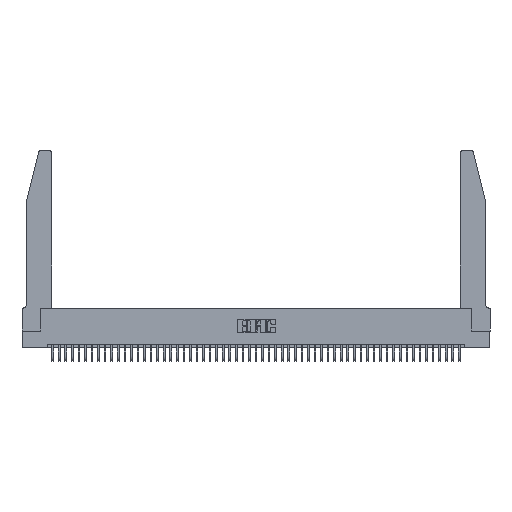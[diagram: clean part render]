
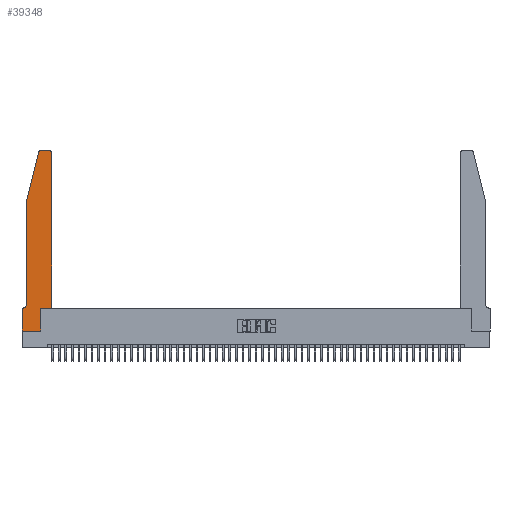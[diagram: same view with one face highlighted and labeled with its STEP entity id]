
A CAD part, top view. The second image highlights one B-rep face of the part: STEP entity #39348.
In plain terms, the highlighted planar face has unit normal (0, 0, 1).
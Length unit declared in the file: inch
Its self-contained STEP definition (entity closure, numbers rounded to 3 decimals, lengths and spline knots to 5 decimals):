
#161 = LINE ( 'NONE', #11159, #33100 ) ;
#1944 = AXIS2_PLACEMENT_3D ( 'NONE', #32347, #7744, #36463 ) ;
#1962 = CARTESIAN_POINT ( 'NONE',  ( 0.0755, 0.35, 0.37 ) ) ;
#2098 = ORIENTED_EDGE ( 'NONE', *, *, #39036, .T. ) ;
#2724 = VECTOR ( 'NONE', #28779, 39.37008 ) ;
#3052 = CARTESIAN_POINT ( 'NONE',  ( 0.25487, 2.72718, 0.37 ) ) ;
#3639 = ORIENTED_EDGE ( 'NONE', *, *, #39453, .T. ) ;
#4787 = EDGE_CURVE ( 'NONE', #17906, #26428, #24658, .T. ) ;
#5095 = VECTOR ( 'NONE', #18629, 39.37008 ) ;
#5466 = CARTESIAN_POINT ( 'NONE',  ( 0.2865, 0.35, 0.37 ) ) ;
#5664 = VERTEX_POINT ( 'NONE', #5466 ) ;
#6022 = CARTESIAN_POINT ( 'NONE',  ( 0.4505, 0.35, 0.37 ) ) ;
#6706 = EDGE_CURVE ( 'NONE', #15442, #36207, #12952, .T. ) ;
#7058 = ORIENTED_EDGE ( 'NONE', *, *, #6706, .T. ) ;
#7272 = EDGE_CURVE ( 'NONE', #49576, #31790, #52472, .T. ) ;
#7744 = DIRECTION ( 'NONE',  ( 0., 0., 1. ) ) ;
#7848 = VERTEX_POINT ( 'NONE', #42641 ) ;
#8058 = CARTESIAN_POINT ( 'NONE',  ( 0.0755, 2., 0.37 ) ) ;
#8470 = CARTESIAN_POINT ( 'NONE',  ( 0., 0.35, 0.37 ) ) ;
#10152 = DIRECTION ( 'NONE',  ( -1., 0., 0. ) ) ;
#10817 = CARTESIAN_POINT ( 'NONE',  ( 0.4205, 2.72, 0.37 ) ) ;
#11159 = CARTESIAN_POINT ( 'NONE',  ( 0., 0., 0.37 ) ) ;
#12011 = CARTESIAN_POINT ( 'NONE',  ( 0.2605, 2.75, 0.37 ) ) ;
#12945 = VERTEX_POINT ( 'NONE', #38376 ) ;
#12949 = FACE_OUTER_BOUND ( 'NONE', #35322, .T. ) ;
#12952 = CIRCLE ( 'NONE', #1944, 0.03 ) ;
#13462 = DIRECTION ( 'NONE',  ( 0., 0., -1. ) ) ;
#13752 = VECTOR ( 'NONE', #10152, 39.37008 ) ;
#14479 = CARTESIAN_POINT ( 'NONE',  ( 0.4505, 0.35, 0.37 ) ) ;
#14942 = DIRECTION ( 'NONE',  ( 1., 0., 0. ) ) ;
#14978 = CARTESIAN_POINT ( 'NONE',  ( 0.0755, 0.42, 0.37 ) ) ;
#15179 = VERTEX_POINT ( 'NONE', #40753 ) ;
#15194 = EDGE_CURVE ( 'NONE', #15179, #7848, #45308, .T. ) ;
#15442 = VERTEX_POINT ( 'NONE', #46208 ) ;
#15621 = ORIENTED_EDGE ( 'NONE', *, *, #24642, .T. ) ;
#16745 = DIRECTION ( 'NONE',  ( 0., 0., 1. ) ) ;
#16920 = VECTOR ( 'NONE', #31723, 39.37008 ) ;
#17074 = CARTESIAN_POINT ( 'NONE',  ( 0.4505, 0.35, 0.37 ) ) ;
#17879 = EDGE_CURVE ( 'NONE', #12945, #15442, #19549, .T. ) ;
#17906 = VERTEX_POINT ( 'NONE', #8058 ) ;
#18629 = DIRECTION ( 'NONE',  ( 1., 0., 0. ) ) ;
#19549 = LINE ( 'NONE', #12011, #50748 ) ;
#21820 = ORIENTED_EDGE ( 'NONE', *, *, #4787, .T. ) ;
#23249 = VERTEX_POINT ( 'NONE', #42673 ) ;
#23628 = VECTOR ( 'NONE', #32767, 39.37008 ) ;
#24642 = EDGE_CURVE ( 'NONE', #23249, #5664, #49626, .T. ) ;
#24658 = LINE ( 'NONE', #48991, #2724 ) ;
#24697 = LINE ( 'NONE', #1962, #13752 ) ;
#25936 = ORIENTED_EDGE ( 'NONE', *, *, #42427, .T. ) ;
#26428 = VERTEX_POINT ( 'NONE', #14978 ) ;
#26989 = LINE ( 'NONE', #14479, #5095 ) ;
#27139 = CIRCLE ( 'NONE', #40269, 0.03 ) ;
#27840 = LINE ( 'NONE', #39721, #16920 ) ;
#28653 = CARTESIAN_POINT ( 'NONE',  ( 0., 0., 0.37 ) ) ;
#28666 = CARTESIAN_POINT ( 'NONE',  ( 0.4505, 2.72, 0.37 ) ) ;
#28779 = DIRECTION ( 'NONE',  ( 0., -1., 0. ) ) ;
#31723 = DIRECTION ( 'NONE',  ( -0.239, -0.971, 0. ) ) ;
#31790 = VERTEX_POINT ( 'NONE', #28666 ) ;
#32347 = CARTESIAN_POINT ( 'NONE',  ( 0.284, 2.72, 0.37 ) ) ;
#32767 = DIRECTION ( 'NONE',  ( 0., -1., 0. ) ) ;
#32853 = ORIENTED_EDGE ( 'NONE', *, *, #49271, .T. ) ;
#33100 = VECTOR ( 'NONE', #35755, 39.37008 ) ;
#33589 = ORIENTED_EDGE ( 'NONE', *, *, #50403, .T. ) ;
#34962 = DIRECTION ( 'NONE',  ( 0., 1., 0. ) ) ;
#35322 = EDGE_LOOP ( 'NONE', ( #40815, #7058, #25936, #21820, #3639, #33589, #37766, #32853, #15621, #40193, #40201, #2098 ) ) ;
#35755 = DIRECTION ( 'NONE',  ( 1., 0., 0. ) ) ;
#36051 = VECTOR ( 'NONE', #34962, 39.37008 ) ;
#36207 = VERTEX_POINT ( 'NONE', #3052 ) ;
#36362 = VECTOR ( 'NONE', #46972, 39.37008 ) ;
#36463 = DIRECTION ( 'NONE',  ( 1., 0., 0. ) ) ;
#37112 = CARTESIAN_POINT ( 'NONE',  ( 0.0055, 0.35, 0.37 ) ) ;
#37766 = ORIENTED_EDGE ( 'NONE', *, *, #15194, .T. ) ;
#37928 = VERTEX_POINT ( 'NONE', #37112 ) ;
#38020 = CARTESIAN_POINT ( 'NONE',  ( 0.0055, 0.42, 0.37 ) ) ;
#38376 = CARTESIAN_POINT ( 'NONE',  ( 0.4205, 2.75, 0.37 ) ) ;
#39036 = EDGE_CURVE ( 'NONE', #31790, #12945, #27139, .T. ) ;
#39260 = AXIS2_PLACEMENT_3D ( 'NONE', #8470, #16745, #45292 ) ;
#39348 = ADVANCED_FACE ( 'NONE', ( #12949 ), #41226, .T. ) ;
#39453 = EDGE_CURVE ( 'NONE', #26428, #37928, #48720, .T. ) ;
#39503 = DIRECTION ( 'NONE',  ( 0., 0., 1. ) ) ;
#39721 = CARTESIAN_POINT ( 'NONE',  ( 0.0755, 2., 0.37 ) ) ;
#40193 = ORIENTED_EDGE ( 'NONE', *, *, #40445, .T. ) ;
#40201 = ORIENTED_EDGE ( 'NONE', *, *, #7272, .T. ) ;
#40269 = AXIS2_PLACEMENT_3D ( 'NONE', #10817, #39503, #14942 ) ;
#40445 = EDGE_CURVE ( 'NONE', #5664, #49576, #26989, .T. ) ;
#40753 = CARTESIAN_POINT ( 'NONE',  ( 0., 0.35, 0.37 ) ) ;
#40815 = ORIENTED_EDGE ( 'NONE', *, *, #17879, .T. ) ;
#41226 = PLANE ( 'NONE',  #39260 ) ;
#42072 = DIRECTION ( 'NONE',  ( -1., 0., 0. ) ) ;
#42427 = EDGE_CURVE ( 'NONE', #36207, #17906, #27840, .T. ) ;
#42641 = CARTESIAN_POINT ( 'NONE',  ( 0., 0., 0.37 ) ) ;
#42673 = CARTESIAN_POINT ( 'NONE',  ( 0.2865, 0., 0.37 ) ) ;
#42905 = CARTESIAN_POINT ( 'NONE',  ( 0.2865, 0.35, 0.37 ) ) ;
#44673 = AXIS2_PLACEMENT_3D ( 'NONE', #38020, #13462, #42072 ) ;
#45292 = DIRECTION ( 'NONE',  ( 1., 0., 0. ) ) ;
#45308 = LINE ( 'NONE', #28653, #23628 ) ;
#46208 = CARTESIAN_POINT ( 'NONE',  ( 0.284, 2.75, 0.37 ) ) ;
#46972 = DIRECTION ( 'NONE',  ( 0., 1., 0. ) ) ;
#48720 = CIRCLE ( 'NONE', #44673, 0.07 ) ;
#48991 = CARTESIAN_POINT ( 'NONE',  ( 0.0755, 2., 0.37 ) ) ;
#49271 = EDGE_CURVE ( 'NONE', #7848, #23249, #161, .T. ) ;
#49576 = VERTEX_POINT ( 'NONE', #17074 ) ;
#49626 = LINE ( 'NONE', #42905, #36362 ) ;
#50403 = EDGE_CURVE ( 'NONE', #37928, #15179, #24697, .T. ) ;
#50748 = VECTOR ( 'NONE', #52652, 39.37008 ) ;
#52472 = LINE ( 'NONE', #6022, #36051 ) ;
#52652 = DIRECTION ( 'NONE',  ( -1., 0., 0. ) ) ;
